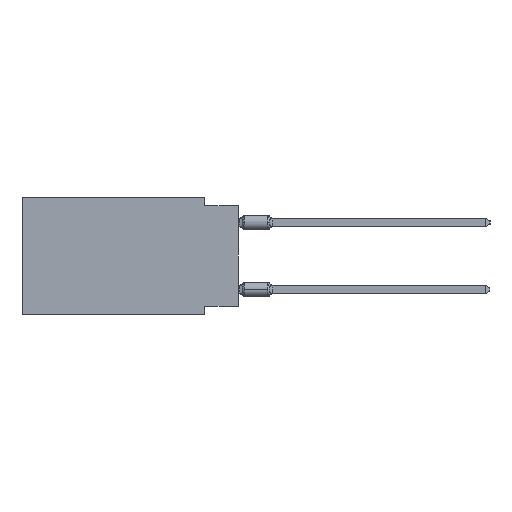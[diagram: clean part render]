
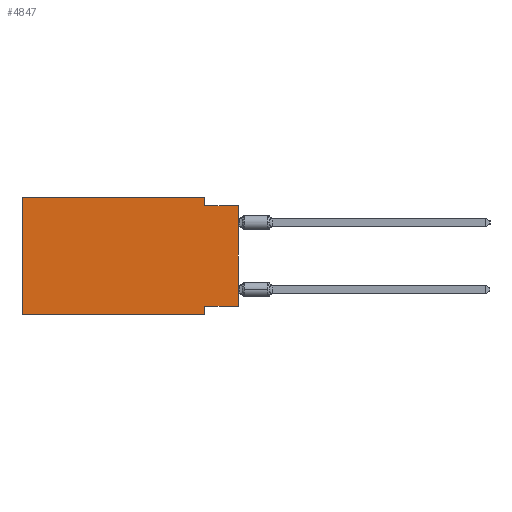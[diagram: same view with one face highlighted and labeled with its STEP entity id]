
A CAD part, left-side view. The second image highlights one B-rep face of the part: STEP entity #4847.
In plain terms, the highlighted planar face has unit normal (-1, 0, 0).
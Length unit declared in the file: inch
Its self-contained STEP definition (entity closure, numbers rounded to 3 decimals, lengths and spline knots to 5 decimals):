
#19 = ORIENTED_EDGE ( 'NONE', *, *, #31560, .F. ) ;
#130 = DIRECTION ( 'NONE',  ( 0., 0., 1. ) ) ;
#761 = CARTESIAN_POINT ( 'NONE',  ( 0., 0.645, 0. ) ) ;
#2625 = CARTESIAN_POINT ( 'NONE',  ( 0., 0., -0.325 ) ) ;
#3795 = EDGE_CURVE ( 'NONE', #12297, #24135, #44640, .T. ) ;
#4147 = CARTESIAN_POINT ( 'NONE',  ( 0., 0., 0. ) ) ;
#4847 = ADVANCED_FACE ( 'NONE', ( #17489 ), #14234, .F. ) ;
#6419 = LINE ( 'NONE', #2625, #51330 ) ;
#6976 = ORIENTED_EDGE ( 'NONE', *, *, #41359, .T. ) ;
#8148 = CARTESIAN_POINT ( 'NONE',  ( 0., 0.645, 0. ) ) ;
#8810 = ORIENTED_EDGE ( 'NONE', *, *, #3795, .F. ) ;
#9141 = DIRECTION ( 'NONE',  ( 0., 0., -1. ) ) ;
#9250 = VECTOR ( 'NONE', #14912, 39.37008 ) ;
#11584 = DIRECTION ( 'NONE',  ( 0., 0., -1. ) ) ;
#12297 = VERTEX_POINT ( 'NONE', #41352 ) ;
#12874 = CARTESIAN_POINT ( 'NONE',  ( 0., 0.645, -0.35 ) ) ;
#13551 = EDGE_CURVE ( 'NONE', #14263, #30756, #49360, .T. ) ;
#14234 = PLANE ( 'NONE',  #52039 ) ;
#14263 = VERTEX_POINT ( 'NONE', #42842 ) ;
#14716 = DIRECTION ( 'NONE',  ( 0., -1., 0. ) ) ;
#14912 = DIRECTION ( 'NONE',  ( 0., -1., 0. ) ) ;
#15626 = DIRECTION ( 'NONE',  ( 0., 0., -1. ) ) ;
#15672 = EDGE_CURVE ( 'NONE', #48870, #24135, #31384, .T. ) ;
#17216 = DIRECTION ( 'NONE',  ( 1., 0., 0. ) ) ;
#17489 = FACE_OUTER_BOUND ( 'NONE', #19806, .T. ) ;
#18314 = CARTESIAN_POINT ( 'NONE',  ( 0., 0., -0.025 ) ) ;
#19058 = DIRECTION ( 'NONE',  ( 0., 1., 0. ) ) ;
#19174 = CARTESIAN_POINT ( 'NONE',  ( 0., 0.1, 0. ) ) ;
#19806 = EDGE_LOOP ( 'NONE', ( #6976, #35035, #19, #25022, #38232, #28060, #8810, #21274 ) ) ;
#20050 = LINE ( 'NONE', #4147, #31524 ) ;
#20236 = LINE ( 'NONE', #48133, #49959 ) ;
#21274 = ORIENTED_EDGE ( 'NONE', *, *, #22617, .F. ) ;
#22470 = EDGE_CURVE ( 'NONE', #27872, #52224, #34106, .T. ) ;
#22617 = EDGE_CURVE ( 'NONE', #25431, #12297, #6419, .T. ) ;
#23446 = CARTESIAN_POINT ( 'NONE',  ( 0., 0.1, -0.35 ) ) ;
#24135 = VERTEX_POINT ( 'NONE', #32461 ) ;
#25022 = ORIENTED_EDGE ( 'NONE', *, *, #22470, .F. ) ;
#25431 = VERTEX_POINT ( 'NONE', #48285 ) ;
#27872 = VERTEX_POINT ( 'NONE', #8148 ) ;
#28060 = ORIENTED_EDGE ( 'NONE', *, *, #15672, .T. ) ;
#30376 = VECTOR ( 'NONE', #14716, 39.37008 ) ;
#30756 = VERTEX_POINT ( 'NONE', #18314 ) ;
#31384 = LINE ( 'NONE', #35425, #30376 ) ;
#31524 = VECTOR ( 'NONE', #130, 39.37008 ) ;
#31560 = EDGE_CURVE ( 'NONE', #52224, #14263, #44124, .T. ) ;
#32461 = CARTESIAN_POINT ( 'NONE',  ( 0., 0.1, -0.35 ) ) ;
#33877 = CARTESIAN_POINT ( 'NONE',  ( 0., 0.645, 0. ) ) ;
#34106 = LINE ( 'NONE', #761, #9250 ) ;
#35035 = ORIENTED_EDGE ( 'NONE', *, *, #13551, .F. ) ;
#35425 = CARTESIAN_POINT ( 'NONE',  ( 0., 0.645, -0.35 ) ) ;
#35827 = DIRECTION ( 'NONE',  ( 0., 0., 1. ) ) ;
#38232 = ORIENTED_EDGE ( 'NONE', *, *, #48263, .F. ) ;
#41047 = CARTESIAN_POINT ( 'NONE',  ( 0., 0., -0.025 ) ) ;
#41352 = CARTESIAN_POINT ( 'NONE',  ( 0., 0.1, -0.325 ) ) ;
#41359 = EDGE_CURVE ( 'NONE', #25431, #30756, #20050, .T. ) ;
#42242 = VECTOR ( 'NONE', #53128, 39.37008 ) ;
#42842 = CARTESIAN_POINT ( 'NONE',  ( 0., 0.1, -0.025 ) ) ;
#44124 = LINE ( 'NONE', #48118, #50809 ) ;
#44640 = LINE ( 'NONE', #23446, #49414 ) ;
#48118 = CARTESIAN_POINT ( 'NONE',  ( 0., 0.1, 0. ) ) ;
#48133 = CARTESIAN_POINT ( 'NONE',  ( 0., 0.645, 0. ) ) ;
#48263 = EDGE_CURVE ( 'NONE', #48870, #27872, #20236, .T. ) ;
#48285 = CARTESIAN_POINT ( 'NONE',  ( 0., 0., -0.325 ) ) ;
#48870 = VERTEX_POINT ( 'NONE', #12874 ) ;
#49360 = LINE ( 'NONE', #41047, #42242 ) ;
#49414 = VECTOR ( 'NONE', #11584, 39.37008 ) ;
#49959 = VECTOR ( 'NONE', #35827, 39.37008 ) ;
#50809 = VECTOR ( 'NONE', #15626, 39.37008 ) ;
#51330 = VECTOR ( 'NONE', #19058, 39.37008 ) ;
#52039 = AXIS2_PLACEMENT_3D ( 'NONE', #33877, #17216, #9141 ) ;
#52224 = VERTEX_POINT ( 'NONE', #19174 ) ;
#53128 = DIRECTION ( 'NONE',  ( 0., -1., 0. ) ) ;
